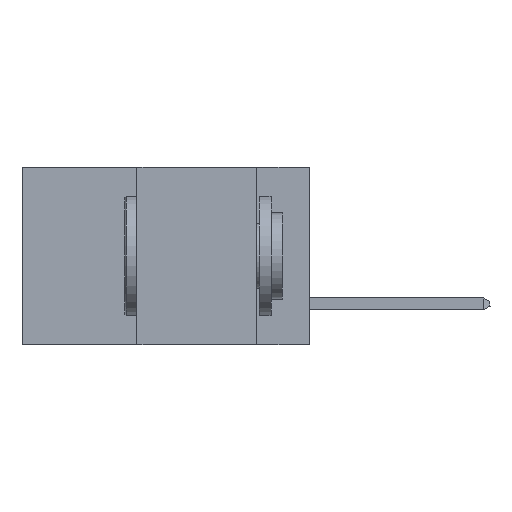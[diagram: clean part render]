
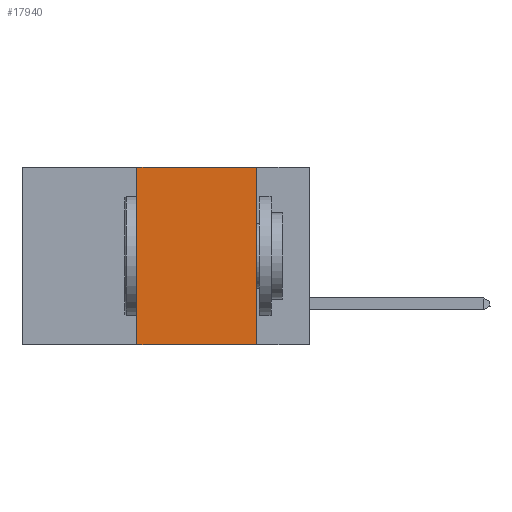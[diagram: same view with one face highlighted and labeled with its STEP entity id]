
A CAD part, left-side view. The second image highlights one B-rep face of the part: STEP entity #17940.
In plain terms, the highlighted planar face has unit normal (-1, 0, 0).
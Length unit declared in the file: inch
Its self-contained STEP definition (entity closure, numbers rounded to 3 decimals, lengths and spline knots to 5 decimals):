
#1892 = EDGE_LOOP ( 'NONE', ( #20855, #6758, #2003, #19827 ) ) ;
#2003 = ORIENTED_EDGE ( 'NONE', *, *, #15137, .F. ) ;
#2032 = VERTEX_POINT ( 'NONE', #16364 ) ;
#3847 = LINE ( 'NONE', #10880, #11639 ) ;
#4662 = VERTEX_POINT ( 'NONE', #8834 ) ;
#5968 = AXIS2_PLACEMENT_3D ( 'NONE', #18425, #10216, #24667 ) ;
#6758 = ORIENTED_EDGE ( 'NONE', *, *, #17664, .F. ) ;
#8200 = CARTESIAN_POINT ( 'NONE',  ( 0., 0.36, -0.37 ) ) ;
#8834 = CARTESIAN_POINT ( 'NONE',  ( 0., 0.11, 0. ) ) ;
#10216 = DIRECTION ( 'NONE',  ( 1., 0., 0. ) ) ;
#10544 = FACE_OUTER_BOUND ( 'NONE', #1892, .T. ) ;
#10585 = DIRECTION ( 'NONE',  ( 0., -1., 0. ) ) ;
#10880 = CARTESIAN_POINT ( 'NONE',  ( 0., 0.6, -0.37 ) ) ;
#10902 = EDGE_CURVE ( 'NONE', #4662, #13739, #17121, .T. ) ;
#11010 = LINE ( 'NONE', #20031, #12637 ) ;
#11216 = VECTOR ( 'NONE', #10585, 39.37008 ) ;
#11639 = VECTOR ( 'NONE', #25254, 39.37008 ) ;
#11949 = CARTESIAN_POINT ( 'NONE',  ( 0., 0.11, 0. ) ) ;
#12637 = VECTOR ( 'NONE', #19943, 39.37008 ) ;
#13739 = VERTEX_POINT ( 'NONE', #21976 ) ;
#14840 = CARTESIAN_POINT ( 'NONE',  ( 0., 0.6, 0. ) ) ;
#15137 = EDGE_CURVE ( 'NONE', #18939, #2032, #11010, .T. ) ;
#16364 = CARTESIAN_POINT ( 'NONE',  ( 0., 0.36, 0. ) ) ;
#17121 = LINE ( 'NONE', #11949, #21013 ) ;
#17664 = EDGE_CURVE ( 'NONE', #2032, #4662, #25129, .T. ) ;
#17940 = ADVANCED_FACE ( 'NONE', ( #10544 ), #18603, .F. ) ;
#18425 = CARTESIAN_POINT ( 'NONE',  ( 0., 0.6, 0. ) ) ;
#18603 = PLANE ( 'NONE',  #5968 ) ;
#18939 = VERTEX_POINT ( 'NONE', #8200 ) ;
#19827 = ORIENTED_EDGE ( 'NONE', *, *, #22635, .T. ) ;
#19943 = DIRECTION ( 'NONE',  ( 0., 0., 1. ) ) ;
#20031 = CARTESIAN_POINT ( 'NONE',  ( 0., 0.36, 0. ) ) ;
#20153 = DIRECTION ( 'NONE',  ( 0., 0., -1. ) ) ;
#20855 = ORIENTED_EDGE ( 'NONE', *, *, #10902, .F. ) ;
#21013 = VECTOR ( 'NONE', #20153, 39.37008 ) ;
#21976 = CARTESIAN_POINT ( 'NONE',  ( 0., 0.11, -0.37 ) ) ;
#22635 = EDGE_CURVE ( 'NONE', #18939, #13739, #3847, .T. ) ;
#24667 = DIRECTION ( 'NONE',  ( 0., 0., -1. ) ) ;
#25129 = LINE ( 'NONE', #14840, #11216 ) ;
#25254 = DIRECTION ( 'NONE',  ( 0., -1., 0. ) ) ;
